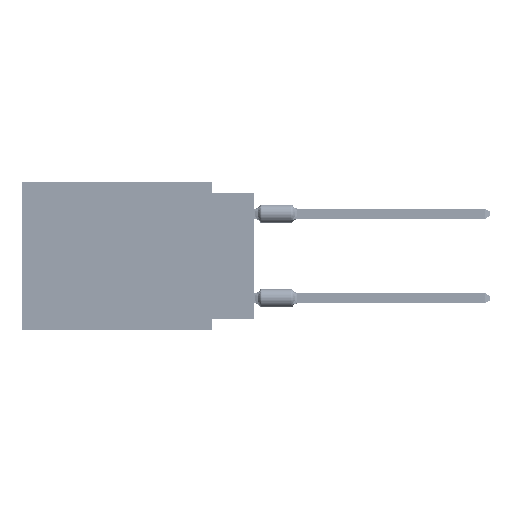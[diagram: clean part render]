
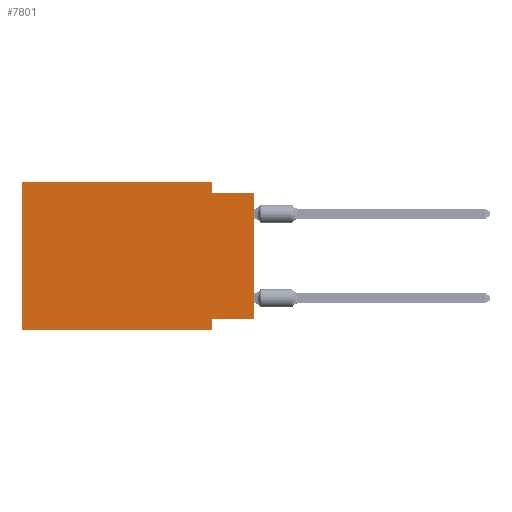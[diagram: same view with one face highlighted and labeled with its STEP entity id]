
A CAD part, left-side view. The second image highlights one B-rep face of the part: STEP entity #7801.
In plain terms, the highlighted planar face has unit normal (-1, 0, 0).
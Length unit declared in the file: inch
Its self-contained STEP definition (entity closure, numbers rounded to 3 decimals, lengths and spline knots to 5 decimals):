
#310 = LINE ( 'NONE', #7814, #14933 ) ;
#1118 = ORIENTED_EDGE ( 'NONE', *, *, #1742, .F. ) ;
#1742 = EDGE_CURVE ( 'NONE', #34046, #13353, #7013, .T. ) ;
#2046 = CARTESIAN_POINT ( 'NONE',  ( 0., 0.1, -0.35 ) ) ;
#2434 = DIRECTION ( 'NONE',  ( 0., -1., 0. ) ) ;
#5643 = VERTEX_POINT ( 'NONE', #14281 ) ;
#6849 = LINE ( 'NONE', #70210, #37910 ) ;
#6971 = DIRECTION ( 'NONE',  ( 0., -1., 0. ) ) ;
#7013 = LINE ( 'NONE', #24915, #54410 ) ;
#7801 = ADVANCED_FACE ( 'NONE', ( #9597 ), #53996, .F. ) ;
#7808 = LINE ( 'NONE', #58566, #22395 ) ;
#7814 = CARTESIAN_POINT ( 'NONE',  ( 0., 0.55, 0. ) ) ;
#9597 = FACE_OUTER_BOUND ( 'NONE', #76497, .T. ) ;
#13353 = VERTEX_POINT ( 'NONE', #18379 ) ;
#14281 = CARTESIAN_POINT ( 'NONE',  ( 0., 0.1, -0.35 ) ) ;
#14933 = VECTOR ( 'NONE', #38720, 39.37008 ) ;
#15193 = LINE ( 'NONE', #78432, #60576 ) ;
#15450 = ORIENTED_EDGE ( 'NONE', *, *, #30902, .F. ) ;
#15904 = LINE ( 'NONE', #46622, #79443 ) ;
#17074 = EDGE_CURVE ( 'NONE', #43689, #38463, #15904, .T. ) ;
#18379 = CARTESIAN_POINT ( 'NONE',  ( 0., 0.55, 0. ) ) ;
#21021 = CARTESIAN_POINT ( 'NONE',  ( 0., 0., -0.325 ) ) ;
#21591 = ORIENTED_EDGE ( 'NONE', *, *, #27311, .T. ) ;
#21894 = VERTEX_POINT ( 'NONE', #21021 ) ;
#22395 = VECTOR ( 'NONE', #64983, 39.37008 ) ;
#22414 = VECTOR ( 'NONE', #6971, 39.37008 ) ;
#23263 = DIRECTION ( 'NONE',  ( 1., 0., 0. ) ) ;
#24915 = CARTESIAN_POINT ( 'NONE',  ( 0., 0.55, 0. ) ) ;
#27311 = EDGE_CURVE ( 'NONE', #34046, #5643, #53276, .T. ) ;
#29289 = DIRECTION ( 'NONE',  ( 0., 1., 0. ) ) ;
#30902 = EDGE_CURVE ( 'NONE', #21894, #78841, #15193, .T. ) ;
#32987 = DIRECTION ( 'NONE',  ( 0., 0., -1. ) ) ;
#33125 = ORIENTED_EDGE ( 'NONE', *, *, #45333, .F. ) ;
#34046 = VERTEX_POINT ( 'NONE', #50989 ) ;
#35361 = CARTESIAN_POINT ( 'NONE',  ( 0., 0., -0.025 ) ) ;
#37311 = ORIENTED_EDGE ( 'NONE', *, *, #47790, .F. ) ;
#37513 = CARTESIAN_POINT ( 'NONE',  ( 0., 0.1, -0.025 ) ) ;
#37910 = VECTOR ( 'NONE', #2434, 39.37008 ) ;
#37985 = EDGE_CURVE ( 'NONE', #78841, #5643, #61072, .T. ) ;
#38463 = VERTEX_POINT ( 'NONE', #37513 ) ;
#38720 = DIRECTION ( 'NONE',  ( 0., -1., 0. ) ) ;
#43689 = VERTEX_POINT ( 'NONE', #75010 ) ;
#45333 = EDGE_CURVE ( 'NONE', #38463, #61599, #6849, .T. ) ;
#46622 = CARTESIAN_POINT ( 'NONE',  ( 0., 0.1, 0. ) ) ;
#47250 = CARTESIAN_POINT ( 'NONE',  ( 0., 0.1, -0.325 ) ) ;
#47790 = EDGE_CURVE ( 'NONE', #13353, #43689, #310, .T. ) ;
#50248 = CARTESIAN_POINT ( 'NONE',  ( 0., 0.55, -0.35 ) ) ;
#50989 = CARTESIAN_POINT ( 'NONE',  ( 0., 0.55, -0.35 ) ) ;
#51276 = AXIS2_PLACEMENT_3D ( 'NONE', #60200, #23263, #66365 ) ;
#52827 = DIRECTION ( 'NONE',  ( 0., 0., -1. ) ) ;
#53276 = LINE ( 'NONE', #50248, #22414 ) ;
#53996 = PLANE ( 'NONE',  #51276 ) ;
#54410 = VECTOR ( 'NONE', #67973, 39.37008 ) ;
#54542 = ORIENTED_EDGE ( 'NONE', *, *, #74220, .T. ) ;
#54883 = ORIENTED_EDGE ( 'NONE', *, *, #17074, .F. ) ;
#58566 = CARTESIAN_POINT ( 'NONE',  ( 0., 0., 0. ) ) ;
#60200 = CARTESIAN_POINT ( 'NONE',  ( 0., 0.55, 0. ) ) ;
#60576 = VECTOR ( 'NONE', #29289, 39.37008 ) ;
#61072 = LINE ( 'NONE', #2046, #77343 ) ;
#61599 = VERTEX_POINT ( 'NONE', #35361 ) ;
#64298 = ORIENTED_EDGE ( 'NONE', *, *, #37985, .F. ) ;
#64983 = DIRECTION ( 'NONE',  ( 0., 0., 1. ) ) ;
#66365 = DIRECTION ( 'NONE',  ( 0., 0., -1. ) ) ;
#67973 = DIRECTION ( 'NONE',  ( 0., 0., 1. ) ) ;
#70210 = CARTESIAN_POINT ( 'NONE',  ( 0., 0., -0.025 ) ) ;
#74220 = EDGE_CURVE ( 'NONE', #21894, #61599, #7808, .T. ) ;
#75010 = CARTESIAN_POINT ( 'NONE',  ( 0., 0.1, 0. ) ) ;
#76497 = EDGE_LOOP ( 'NONE', ( #54542, #33125, #54883, #37311, #1118, #21591, #64298, #15450 ) ) ;
#77343 = VECTOR ( 'NONE', #32987, 39.37008 ) ;
#78432 = CARTESIAN_POINT ( 'NONE',  ( 0., 0., -0.325 ) ) ;
#78841 = VERTEX_POINT ( 'NONE', #47250 ) ;
#79443 = VECTOR ( 'NONE', #52827, 39.37008 ) ;
